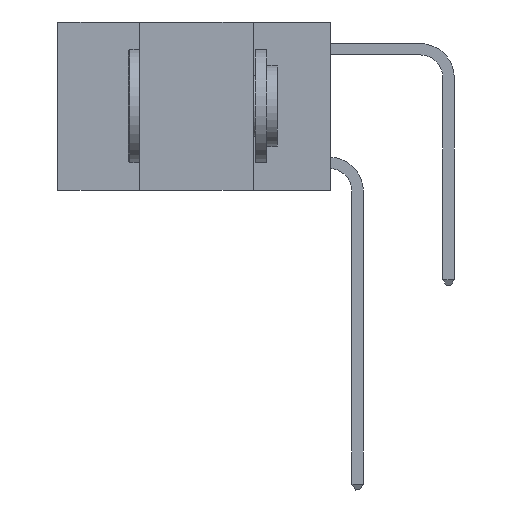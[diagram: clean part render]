
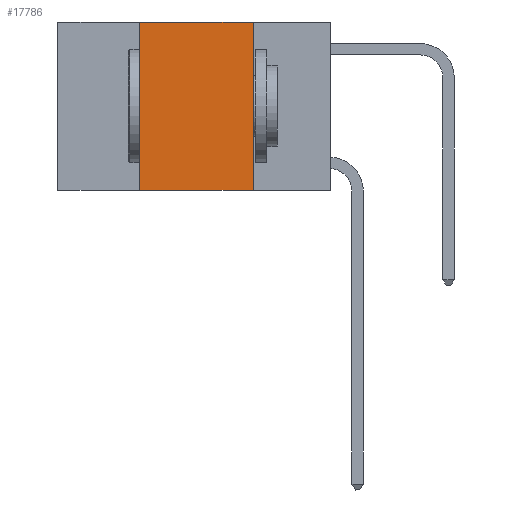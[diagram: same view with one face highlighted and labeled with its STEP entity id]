
A CAD part, left-side view. The second image highlights one B-rep face of the part: STEP entity #17786.
In plain terms, the highlighted planar face has unit normal (-1, 0, 0).
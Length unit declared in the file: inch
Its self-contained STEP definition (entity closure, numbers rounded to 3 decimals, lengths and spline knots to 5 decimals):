
#2 = DIRECTION ( 'NONE',  ( 0., -1., 0. ) ) ;
#777 = CARTESIAN_POINT ( 'NONE',  ( 0., 0.17, 0. ) ) ;
#1543 = CARTESIAN_POINT ( 'NONE',  ( 0., 0.42, 0. ) ) ;
#2118 = DIRECTION ( 'NONE',  ( 0., 0., 1. ) ) ;
#2195 = LINE ( 'NONE', #13656, #11412 ) ;
#2552 = LINE ( 'NONE', #8272, #13595 ) ;
#2765 = EDGE_CURVE ( 'NONE', #7880, #17023, #10491, .T. ) ;
#2786 = VERTEX_POINT ( 'NONE', #7655 ) ;
#2975 = CARTESIAN_POINT ( 'NONE',  ( 0., 0.42, -0.37 ) ) ;
#4242 = ORIENTED_EDGE ( 'NONE', *, *, #5858, .F. ) ;
#4348 = AXIS2_PLACEMENT_3D ( 'NONE', #17051, #9829, #8499 ) ;
#5858 = EDGE_CURVE ( 'NONE', #12250, #2786, #16441, .T. ) ;
#6649 = EDGE_LOOP ( 'NONE', ( #4242, #17882, #15911, #7305 ) ) ;
#7305 = ORIENTED_EDGE ( 'NONE', *, *, #14269, .T. ) ;
#7655 = CARTESIAN_POINT ( 'NONE',  ( 0., 0.17, -0.37 ) ) ;
#7880 = VERTEX_POINT ( 'NONE', #2975 ) ;
#8272 = CARTESIAN_POINT ( 'NONE',  ( 0., 0.6, -0.37 ) ) ;
#8499 = DIRECTION ( 'NONE',  ( 0., 0., -1. ) ) ;
#8676 = FACE_OUTER_BOUND ( 'NONE', #6649, .T. ) ;
#9829 = DIRECTION ( 'NONE',  ( 1., 0., 0. ) ) ;
#10057 = VECTOR ( 'NONE', #2118, 39.37008 ) ;
#10491 = LINE ( 'NONE', #16112, #10057 ) ;
#11217 = EDGE_CURVE ( 'NONE', #17023, #12250, #2195, .T. ) ;
#11345 = PLANE ( 'NONE',  #4348 ) ;
#11412 = VECTOR ( 'NONE', #16467, 39.37008 ) ;
#12250 = VERTEX_POINT ( 'NONE', #16757 ) ;
#12801 = VECTOR ( 'NONE', #15298, 39.37008 ) ;
#13595 = VECTOR ( 'NONE', #2, 39.37008 ) ;
#13656 = CARTESIAN_POINT ( 'NONE',  ( 0., 0.6, 0. ) ) ;
#14269 = EDGE_CURVE ( 'NONE', #7880, #2786, #2552, .T. ) ;
#15298 = DIRECTION ( 'NONE',  ( 0., 0., -1. ) ) ;
#15911 = ORIENTED_EDGE ( 'NONE', *, *, #2765, .F. ) ;
#16112 = CARTESIAN_POINT ( 'NONE',  ( 0., 0.42, 0. ) ) ;
#16441 = LINE ( 'NONE', #777, #12801 ) ;
#16467 = DIRECTION ( 'NONE',  ( 0., -1., 0. ) ) ;
#16757 = CARTESIAN_POINT ( 'NONE',  ( 0., 0.17, 0. ) ) ;
#17023 = VERTEX_POINT ( 'NONE', #1543 ) ;
#17051 = CARTESIAN_POINT ( 'NONE',  ( 0., 0.6, 0. ) ) ;
#17786 = ADVANCED_FACE ( 'NONE', ( #8676 ), #11345, .F. ) ;
#17882 = ORIENTED_EDGE ( 'NONE', *, *, #11217, .F. ) ;
